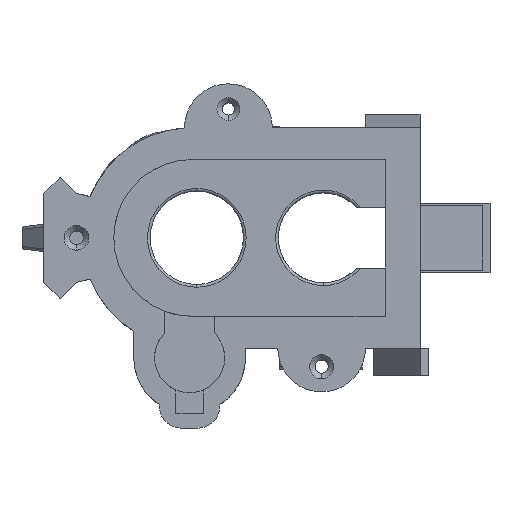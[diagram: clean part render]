
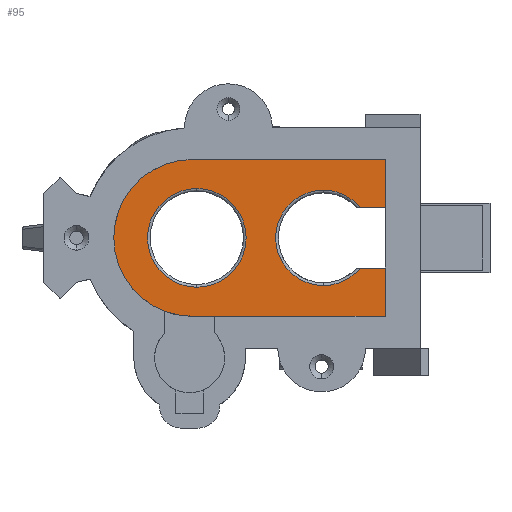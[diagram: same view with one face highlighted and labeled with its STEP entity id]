
A CAD part, left-side view. The second image highlights one B-rep face of the part: STEP entity #95.
In plain terms, the highlighted planar face has unit normal (-1, 0, 0).
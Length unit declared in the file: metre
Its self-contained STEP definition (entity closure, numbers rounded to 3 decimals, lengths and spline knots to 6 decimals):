
#95=ADVANCED_FACE('0:174',(#407,#408,#409),#410,.T.);
#407=FACE_BOUND('',#965,.T.);
#408=FACE_BOUND('',#966,.T.);
#409=FACE_OUTER_BOUND('',#967,.T.);
#410=PLANE('',#968);
#965=EDGE_LOOP('',(#2157,#2158,#2159,#2160,#2161,#2162));
#966=EDGE_LOOP('',(#2163,#2164));
#967=EDGE_LOOP('',(#2165,#2166,#2167,#2168,#2169,#2170,#2171,#2172,#2173,#2174,#2175,#2176,#2177,#2178,#2179,#2180));
#968=AXIS2_PLACEMENT_3D('',#2181,#2182,#2183);
#2157=ORIENTED_EDGE('',*,*,#4230,.T.);
#2158=ORIENTED_EDGE('',*,*,#4234,.T.);
#2159=ORIENTED_EDGE('',*,*,#4232,.T.);
#2160=ORIENTED_EDGE('',*,*,#4235,.F.);
#2161=ORIENTED_EDGE('',*,*,#4218,.F.);
#2162=ORIENTED_EDGE('',*,*,#4214,.F.);
#2163=ORIENTED_EDGE('',*,*,#4081,.F.);
#2164=ORIENTED_EDGE('',*,*,#4236,.F.);
#2165=ORIENTED_EDGE('',*,*,#4237,.F.);
#2166=ORIENTED_EDGE('',*,*,#4238,.F.);
#2167=ORIENTED_EDGE('',*,*,#4239,.F.);
#2168=ORIENTED_EDGE('',*,*,#4240,.F.);
#2169=ORIENTED_EDGE('',*,*,#4241,.F.);
#2170=ORIENTED_EDGE('',*,*,#4242,.T.);
#2171=ORIENTED_EDGE('',*,*,#4243,.T.);
#2172=ORIENTED_EDGE('',*,*,#4244,.T.);
#2173=ORIENTED_EDGE('',*,*,#4245,.F.);
#2174=ORIENTED_EDGE('',*,*,#4246,.F.);
#2175=ORIENTED_EDGE('',*,*,#4247,.T.);
#2176=ORIENTED_EDGE('',*,*,#4248,.F.);
#2177=ORIENTED_EDGE('',*,*,#4249,.F.);
#2178=ORIENTED_EDGE('',*,*,#4250,.F.);
#2179=ORIENTED_EDGE('',*,*,#4251,.T.);
#2180=ORIENTED_EDGE('',*,*,#4252,.F.);
#2181=CARTESIAN_POINT('',(-0.020115,0.057445,0.0));
#2182=DIRECTION('',(-1.0,0.0,0.0));
#2183=DIRECTION('',(0.0,0.0,1.0));
#4081=EDGE_CURVE('0:947',#4819,#4813,#4821,.T.);
#4214=EDGE_CURVE('0:956',#5070,#5065,#5072,.T.);
#4218=EDGE_CURVE('0:956',#5065,#5074,#5079,.T.);
#4230=EDGE_CURVE('3:21217',#5070,#5096,#5098,.T.);
#4232=EDGE_CURVE('3:21256',#5101,#5099,#5102,.T.);
#4234=EDGE_CURVE('3:21262',#5096,#5101,#5104,.T.);
#4235=EDGE_CURVE('0:956',#5074,#5099,#5105,.T.);
#4236=EDGE_CURVE('0:947',#4813,#4819,#5106,.T.);
#4237=EDGE_CURVE('0:1178',#5107,#5108,#5109,.T.);
#4238=EDGE_CURVE('0:1181',#5110,#5107,#5111,.F.);
#4239=EDGE_CURVE('0:1184',#5112,#5110,#5113,.T.);
#4240=EDGE_CURVE('0:1187',#5114,#5112,#5115,.T.);
#4241=EDGE_CURVE('0:1190',#5116,#5114,#5117,.F.);
#4242=EDGE_CURVE('0:1193',#5116,#5118,#5119,.T.);
#4243=EDGE_CURVE('0:1196',#5118,#5120,#5121,.T.);
#4244=EDGE_CURVE('0:1199',#5120,#5122,#5123,.T.);
#4245=EDGE_CURVE('0:1202',#5124,#5122,#5125,.F.);
#4246=EDGE_CURVE('0:1205',#5126,#5124,#5127,.T.);
#4247=EDGE_CURVE('0:1208',#5126,#5128,#5129,.F.);
#4248=EDGE_CURVE('0:1016',#5130,#5128,#5131,.T.);
#4249=EDGE_CURVE('0:1211',#5132,#5130,#5133,.T.);
#4250=EDGE_CURVE('0:1214',#5134,#5132,#5135,.T.);
#4251=EDGE_CURVE('0:1217',#5134,#5136,#5137,.T.);
#4252=EDGE_CURVE('0:1220',#5108,#5136,#5138,.T.);
#4813=VERTEX_POINT('',#6053);
#4819=VERTEX_POINT('',#6059);
#4821=CIRCLE('',#6061,0.009);
#5065=VERTEX_POINT('',#6496);
#5070=VERTEX_POINT('',#6501);
#5072=CIRCLE('',#6542,0.0087);
#5074=VERTEX_POINT('',#6544);
#5079=CIRCLE('',#6549,0.0087);
#5096=VERTEX_POINT('',#6572);
#5098=LINE('',#6575,#6576);
#5099=VERTEX_POINT('',#6577);
#5101=VERTEX_POINT('',#6621);
#5102=LINE('',#6622,#6623);
#5104=LINE('',#6626,#6627);
#5105=CIRCLE('',#6628,0.0087);
#5106=CIRCLE('',#6629,0.009);
#5107=VERTEX_POINT('',#6630);
#5108=VERTEX_POINT('',#6631);
#5109=LINE('',#6632,#6633);
#5110=VERTEX_POINT('',#6634);
#5111=LINE('',#6635,#6636);
#5112=VERTEX_POINT('',#6637);
#5113=LINE('',#6638,#6639);
#5114=VERTEX_POINT('',#6640);
#5115=LINE('',#6641,#6642);
#5116=VERTEX_POINT('',#6643);
#5117=LINE('',#6644,#6645);
#5118=VERTEX_POINT('',#6646);
#5119=LINE('',#6647,#6648);
#5120=VERTEX_POINT('',#6649);
#5121=LINE('',#6650,#6651);
#5122=VERTEX_POINT('',#6652);
#5123=LINE('',#6653,#6654);
#5124=VERTEX_POINT('',#6655);
#5125=LINE('',#6656,#6657);
#5126=VERTEX_POINT('',#6658);
#5127=LINE('',#6659,#6660);
#5128=VERTEX_POINT('',#6661);
#5129=LINE('',#6662,#6663);
#5130=VERTEX_POINT('',#6664);
#5131=B_SPLINE_CURVE_WITH_KNOTS('',3,(#6665,#6666,#6667,#6668,#6669,#6670,#6671,#6672,#6673,#6674,#6675,#6676,#6677,#6678,#6679,#6680),.UNSPECIFIED.,.F.,.F.,(4,3,3,3,3,4),(0.047603,0.054567,0.059611,0.064385,0.074152,0.074835),.UNSPECIFIED.);
#5132=VERTEX_POINT('',#6681);
#5133=LINE('',#6682,#6683);
#5134=VERTEX_POINT('',#6684);
#5135=LINE('',#6685,#6686);
#5136=VERTEX_POINT('',#6687);
#5137=CIRCLE('',#6688,0.0143);
#5138=LINE('',#6689,#6690);
#6053=CARTESIAN_POINT('',(-0.020115,0.0472,-0.009));
#6059=CARTESIAN_POINT('',(-0.020115,0.0472,0.009));
#6061=AXIS2_PLACEMENT_3D('',#8484,#8485,#8486);
#6496=CARTESIAN_POINT('',(-0.020115,0.024119,0.0087));
#6501=CARTESIAN_POINT('',(-0.020115,0.017378,0.0055));
#6542=AXIS2_PLACEMENT_3D('',#8729,#8730,#8731);
#6544=CARTESIAN_POINT('',(-0.020115,0.024119,-0.0087));
#6549=AXIS2_PLACEMENT_3D('',#8741,#8742,#8743);
#6572=CARTESIAN_POINT('',(-0.020115,0.011186,0.005501));
#6575=CARTESIAN_POINT('',(-0.020115,0.036029,0.005499));
#6576=VECTOR('',#8763,1.0);
#6577=CARTESIAN_POINT('',(-0.020115,0.017378,-0.0055));
#6621=CARTESIAN_POINT('',(-0.020115,0.011186,-0.005499));
#6622=CARTESIAN_POINT('',(-0.020115,0.036028,-0.005501));
#6623=VECTOR('',#8764,1.0);
#6626=CARTESIAN_POINT('',(-0.020115,0.011186,0.000002));
#6627=VECTOR('',#8766,1.0);
#6628=AXIS2_PLACEMENT_3D('',#8767,#8768,#8769);
#6629=AXIS2_PLACEMENT_3D('',#8770,#8771,#8772);
#6630=CARTESIAN_POINT('',(-0.020115,0.029178,-0.0201));
#6631=CARTESIAN_POINT('',(-0.020115,0.029178,-0.0143));
#6632=CARTESIAN_POINT('',(-0.020115,0.029178,-0.0201));
#6633=VECTOR('',#8773,1.0);
#6634=CARTESIAN_POINT('',(-0.020115,0.019978,-0.0201));
#6635=CARTESIAN_POINT('',(-0.020115,0.025965,-0.0201));
#6636=VECTOR('',#8774,1.0);
#6637=CARTESIAN_POINT('',(-0.020115,0.019978,-0.0143));
#6638=CARTESIAN_POINT('',(-0.020115,0.019978,-0.0201));
#6639=VECTOR('',#8775,1.0);
#6640=CARTESIAN_POINT('',(-0.020115,0.01284,-0.0143));
#6641=CARTESIAN_POINT('',(-0.020115,0.016409,-0.0143));
#6642=VECTOR('',#8776,1.0);
#6643=CARTESIAN_POINT('',(-0.020115,0.01284,-0.008865));
#6644=CARTESIAN_POINT('',(-0.020115,0.01284,-0.0171));
#6645=VECTOR('',#8777,1.0);
#6646=CARTESIAN_POINT('',(-0.020115,0.006487,-0.008865));
#6647=CARTESIAN_POINT('',(-0.020115,0.013234,-0.008865));
#6648=VECTOR('',#8778,1.0);
#6649=CARTESIAN_POINT('',(-0.020115,0.00649,0.008915));
#6650=CARTESIAN_POINT('',(-0.020115,0.006488,-0.00183));
#6651=VECTOR('',#8779,1.0);
#6652=CARTESIAN_POINT('',(-0.020115,0.01284,0.008915));
#6653=CARTESIAN_POINT('',(-0.020115,0.013234,0.008915));
#6654=VECTOR('',#8780,1.0);
#6655=CARTESIAN_POINT('',(-0.020115,0.01284,0.0143));
#6656=CARTESIAN_POINT('',(-0.020115,0.01284,-0.0171));
#6657=VECTOR('',#8781,1.0);
#6658=CARTESIAN_POINT('',(-0.020115,0.01649,0.0143));
#6659=CARTESIAN_POINT('',(-0.020115,0.034009,0.0143));
#6660=VECTOR('',#8782,1.0);
#6661=CARTESIAN_POINT('',(-0.020115,0.01649,0.0201));
#6662=CARTESIAN_POINT('',(-0.020115,0.01649,-0.000767));
#6663=VECTOR('',#8783,1.0);
#6664=CARTESIAN_POINT('',(-0.020115,0.040076,0.0201));
#6665=CARTESIAN_POINT('',(-0.020115,0.040076,0.0201));
#6666=CARTESIAN_POINT('',(-0.020115,0.038425,0.020101));
#6667=CARTESIAN_POINT('',(-0.020115,0.036624,0.0201));
#6668=CARTESIAN_POINT('',(-0.020115,0.034717,0.0201));
#6669=CARTESIAN_POINT('',(-0.020115,0.033336,0.0201));
#6670=CARTESIAN_POINT('',(-0.020115,0.031899,0.0201));
#6671=CARTESIAN_POINT('',(-0.020115,0.030424,0.0201));
#6672=CARTESIAN_POINT('',(-0.020115,0.029028,0.0201));
#6673=CARTESIAN_POINT('',(-0.020115,0.027598,0.0201));
#6674=CARTESIAN_POINT('',(-0.020115,0.026148,0.0201));
#6675=CARTESIAN_POINT('',(-0.020115,0.023181,0.0201));
#6676=CARTESIAN_POINT('',(-0.020115,0.020131,0.0201));
#6677=CARTESIAN_POINT('',(-0.020115,0.017121,0.0201));
#6678=CARTESIAN_POINT('',(-0.020115,0.016911,0.0201));
#6679=CARTESIAN_POINT('',(-0.020115,0.0167,0.0201));
#6680=CARTESIAN_POINT('',(-0.020115,0.01649,0.0201));
#6681=CARTESIAN_POINT('',(-0.020115,0.040076,0.0143));
#6682=CARTESIAN_POINT('',(-0.020115,0.040076,0.0));
#6683=VECTOR('',#8784,1.0);
#6684=CARTESIAN_POINT('',(-0.020115,0.04804,0.0143));
#6685=CARTESIAN_POINT('',(-0.020115,0.034009,0.0143));
#6686=VECTOR('',#8785,1.0);
#6687=CARTESIAN_POINT('',(-0.020115,0.04804,-0.0143));
#6688=AXIS2_PLACEMENT_3D('',#8786,#8787,#8788);
#6689=CARTESIAN_POINT('',(-0.020115,0.016409,-0.0143));
#6690=VECTOR('',#8789,1.0);
#8484=CARTESIAN_POINT('',(-0.020115,0.0472,0.0));
#8485=DIRECTION('',(-1.0,0.0,0.0));
#8486=DIRECTION('',(0.0,1.0,0.0));
#8729=CARTESIAN_POINT('',(-0.020115,0.024119,0.));
#8730=DIRECTION('',(-1.0,0.0,0.0));
#8731=DIRECTION('',(0.0,1.0,0.0));
#8741=CARTESIAN_POINT('',(-0.020115,0.024119,0.));
#8742=DIRECTION('',(-1.0,0.0,0.0));
#8743=DIRECTION('',(0.0,1.0,0.0));
#8763=DIRECTION('',(0.0,-1.,0.));
#8764=DIRECTION('',(0.0,1.,0.));
#8766=DIRECTION('',(-0.0,0.,-1.));
#8767=CARTESIAN_POINT('',(-0.020115,0.024119,0.));
#8768=DIRECTION('',(-1.0,0.0,0.0));
#8769=DIRECTION('',(0.0,1.0,0.0));
#8770=CARTESIAN_POINT('',(-0.020115,0.0472,0.0));
#8771=DIRECTION('',(-1.0,0.0,0.0));
#8772=DIRECTION('',(0.0,1.0,0.0));
#8773=DIRECTION('',(0.0,0.,1.0));
#8774=DIRECTION('',(-0.0,-1.0,-0.0));
#8775=DIRECTION('',(-0.0,0.,-1.0));
#8776=DIRECTION('',(0.0,1.0,-0.0));
#8777=DIRECTION('',(0.0,0.0,1.0));
#8778=DIRECTION('',(-0.0,-1.0,-0.0));
#8779=DIRECTION('',(0.0,0.,1.));
#8780=DIRECTION('',(0.0,1.0,-0.0));
#8781=DIRECTION('',(0.0,0.0,1.0));
#8782=DIRECTION('',(0.0,-1.0,0.));
#8783=DIRECTION('',(0.0,0.0,-1.0));
#8784=DIRECTION('',(0.0,0.0,1.0));
#8785=DIRECTION('',(0.0,-1.0,0.));
#8786=CARTESIAN_POINT('',(-0.020115,0.04804,0.0));
#8787=DIRECTION('',(-1.0,0.0,0.0));
#8788=DIRECTION('',(0.0,0.0,1.0));
#8789=DIRECTION('',(0.0,1.0,-0.0));
